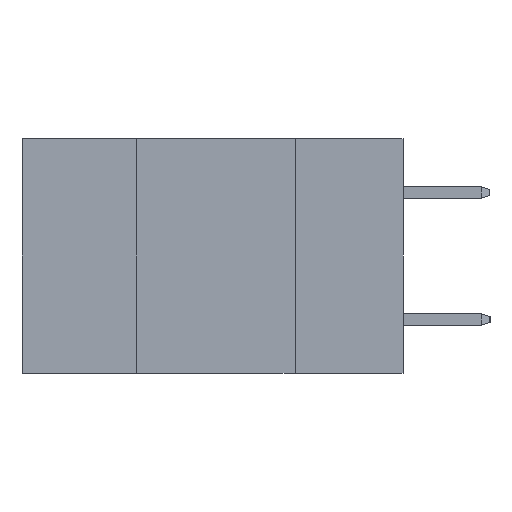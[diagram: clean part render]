
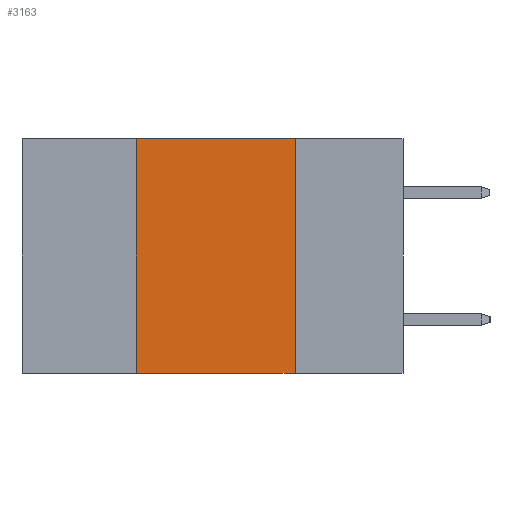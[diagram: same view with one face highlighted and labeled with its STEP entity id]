
A CAD part, left-side view. The second image highlights one B-rep face of the part: STEP entity #3163.
In plain terms, the highlighted planar face has unit normal (-1, 0, 0).
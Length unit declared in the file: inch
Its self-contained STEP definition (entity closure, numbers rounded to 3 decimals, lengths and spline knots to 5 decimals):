
#273 = EDGE_CURVE ( 'NONE', #5346, #9563, #9739, .T. ) ;
#373 = DIRECTION ( 'NONE',  ( 0., -1., 0. ) ) ;
#706 = CARTESIAN_POINT ( 'NONE',  ( 0., 0.6, 0. ) ) ;
#805 = VECTOR ( 'NONE', #7597, 39.37008 ) ;
#1262 = VECTOR ( 'NONE', #8867, 39.37008 ) ;
#1300 = ORIENTED_EDGE ( 'NONE', *, *, #273, .F. ) ;
#1531 = DIRECTION ( 'NONE',  ( 0., -1., 0. ) ) ;
#2305 = CARTESIAN_POINT ( 'NONE',  ( 0., 0.42, -0.37 ) ) ;
#2483 = CARTESIAN_POINT ( 'NONE',  ( 0., 0.17, 0. ) ) ;
#2731 = EDGE_CURVE ( 'NONE', #3820, #5346, #10176, .T. ) ;
#2873 = CARTESIAN_POINT ( 'NONE',  ( 0., 0.42, 0. ) ) ;
#2968 = ORIENTED_EDGE ( 'NONE', *, *, #2731, .F. ) ;
#3025 = CARTESIAN_POINT ( 'NONE',  ( 0., 0.6, 0. ) ) ;
#3163 = ADVANCED_FACE ( 'NONE', ( #8617 ), #7858, .F. ) ;
#3442 = EDGE_LOOP ( 'NONE', ( #1300, #2968, #9906, #7974 ) ) ;
#3820 = VERTEX_POINT ( 'NONE', #2873 ) ;
#3948 = VERTEX_POINT ( 'NONE', #2305 ) ;
#4421 = CARTESIAN_POINT ( 'NONE',  ( 0., 0.6, -0.37 ) ) ;
#4822 = DIRECTION ( 'NONE',  ( 0., 0., -1. ) ) ;
#5270 = CARTESIAN_POINT ( 'NONE',  ( 0., 0.17, -0.37 ) ) ;
#5346 = VERTEX_POINT ( 'NONE', #9995 ) ;
#5880 = EDGE_CURVE ( 'NONE', #3948, #3820, #7503, .T. ) ;
#5991 = LINE ( 'NONE', #4421, #9551 ) ;
#6765 = CARTESIAN_POINT ( 'NONE',  ( 0., 0.42, 0. ) ) ;
#7078 = DIRECTION ( 'NONE',  ( 1., 0., 0. ) ) ;
#7503 = LINE ( 'NONE', #6765, #805 ) ;
#7597 = DIRECTION ( 'NONE',  ( 0., 0., 1. ) ) ;
#7858 = PLANE ( 'NONE',  #8116 ) ;
#7974 = ORIENTED_EDGE ( 'NONE', *, *, #8969, .T. ) ;
#8116 = AXIS2_PLACEMENT_3D ( 'NONE', #706, #7078, #4822 ) ;
#8617 = FACE_OUTER_BOUND ( 'NONE', #3442, .T. ) ;
#8867 = DIRECTION ( 'NONE',  ( 0., 0., -1. ) ) ;
#8969 = EDGE_CURVE ( 'NONE', #3948, #9563, #5991, .T. ) ;
#9107 = VECTOR ( 'NONE', #1531, 39.37008 ) ;
#9551 = VECTOR ( 'NONE', #373, 39.37008 ) ;
#9563 = VERTEX_POINT ( 'NONE', #5270 ) ;
#9739 = LINE ( 'NONE', #2483, #1262 ) ;
#9906 = ORIENTED_EDGE ( 'NONE', *, *, #5880, .F. ) ;
#9995 = CARTESIAN_POINT ( 'NONE',  ( 0., 0.17, 0. ) ) ;
#10176 = LINE ( 'NONE', #3025, #9107 ) ;
